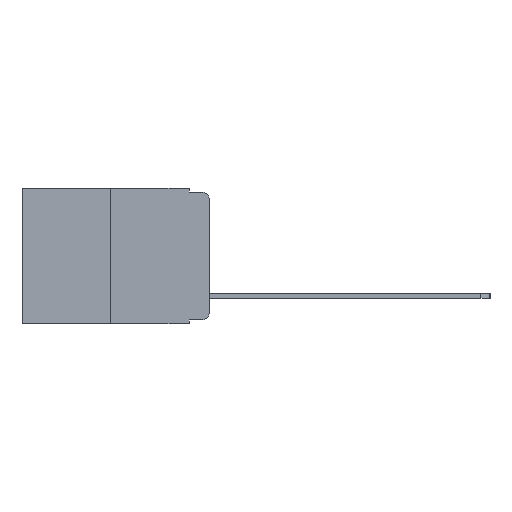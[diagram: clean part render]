
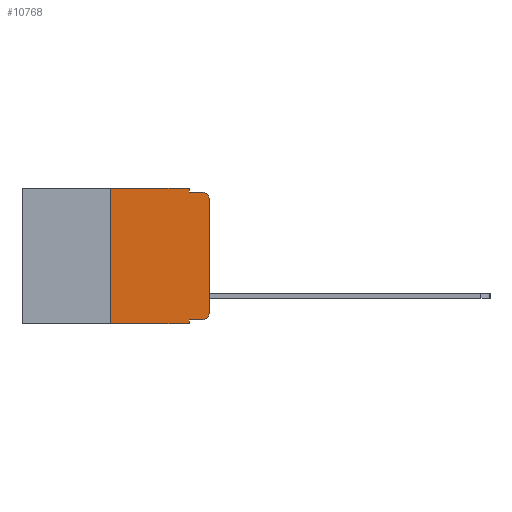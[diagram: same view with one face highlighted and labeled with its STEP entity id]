
A CAD part, left-side view. The second image highlights one B-rep face of the part: STEP entity #10768.
In plain terms, the highlighted planar face has unit normal (-1, 0, 0).
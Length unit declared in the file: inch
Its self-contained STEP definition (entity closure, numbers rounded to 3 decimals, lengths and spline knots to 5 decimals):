
#59 = EDGE_LOOP ( 'NONE', ( #7966, #12042, #20362, #16670, #18114, #4457, #2379, #17849, #21247, #2677 ) ) ;
#522 = CARTESIAN_POINT ( 'NONE',  ( 0., 0.25, -0.343 ) ) ;
#590 = CIRCLE ( 'NONE', #12441, 0.02 ) ;
#1751 = VERTEX_POINT ( 'NONE', #12122 ) ;
#2349 = VERTEX_POINT ( 'NONE', #16459 ) ;
#2371 = DIRECTION ( 'NONE',  ( 0., -1., 0. ) ) ;
#2379 = ORIENTED_EDGE ( 'NONE', *, *, #17304, .T. ) ;
#2425 = VERTEX_POINT ( 'NONE', #12521 ) ;
#2677 = ORIENTED_EDGE ( 'NONE', *, *, #8130, .T. ) ;
#2835 = EDGE_CURVE ( 'NONE', #20767, #2425, #19707, .T. ) ;
#3055 = CARTESIAN_POINT ( 'NONE',  ( 0., 0.02, -0.03 ) ) ;
#3078 = EDGE_CURVE ( 'NONE', #16209, #1751, #15110, .T. ) ;
#3183 = LINE ( 'NONE', #14919, #12591 ) ;
#3663 = VECTOR ( 'NONE', #22484, 39.37008 ) ;
#4039 = CARTESIAN_POINT ( 'NONE',  ( 0., 0.473, -0.343 ) ) ;
#4457 = ORIENTED_EDGE ( 'NONE', *, *, #2835, .F. ) ;
#4600 = CARTESIAN_POINT ( 'NONE',  ( 0., 0.051, -0.343 ) ) ;
#4985 = DIRECTION ( 'NONE',  ( 0., 0., -1. ) ) ;
#5203 = FACE_OUTER_BOUND ( 'NONE', #59, .T. ) ;
#6213 = DIRECTION ( 'NONE',  ( 0., 0., 1. ) ) ;
#6224 = EDGE_CURVE ( 'NONE', #16209, #16141, #14767, .T. ) ;
#6376 = VECTOR ( 'NONE', #8474, 39.37008 ) ;
#7515 = LINE ( 'NONE', #13726, #12458 ) ;
#7887 = AXIS2_PLACEMENT_3D ( 'NONE', #3055, #16147, #4985 ) ;
#7966 = ORIENTED_EDGE ( 'NONE', *, *, #11653, .T. ) ;
#8130 = EDGE_CURVE ( 'NONE', #1751, #2349, #590, .T. ) ;
#8420 = CARTESIAN_POINT ( 'NONE',  ( 0., 0., 0. ) ) ;
#8424 = VERTEX_POINT ( 'NONE', #8442 ) ;
#8442 = CARTESIAN_POINT ( 'NONE',  ( 0., 0.051, 0. ) ) ;
#8474 = DIRECTION ( 'NONE',  ( 0., -1., 0. ) ) ;
#8501 = DIRECTION ( 'NONE',  ( 0., 0., -1. ) ) ;
#8521 = VECTOR ( 'NONE', #2371, 39.37008 ) ;
#8726 = EDGE_CURVE ( 'NONE', #8424, #23268, #3183, .T. ) ;
#8734 = LINE ( 'NONE', #8420, #22222 ) ;
#8911 = EDGE_CURVE ( 'NONE', #23268, #14359, #23161, .T. ) ;
#9411 = CIRCLE ( 'NONE', #7887, 0.02 ) ;
#9768 = CARTESIAN_POINT ( 'NONE',  ( 0., 0.051, -0.01 ) ) ;
#9835 = VERTEX_POINT ( 'NONE', #23696 ) ;
#10120 = CARTESIAN_POINT ( 'NONE',  ( 0., 0.02, -0.313 ) ) ;
#10267 = PLANE ( 'NONE',  #13579 ) ;
#10768 = ADVANCED_FACE ( 'NONE', ( #5203 ), #10267, .F. ) ;
#11653 = EDGE_CURVE ( 'NONE', #2349, #9835, #8734, .T. ) ;
#12000 = DIRECTION ( 'NONE',  ( 0., 0., -1. ) ) ;
#12042 = ORIENTED_EDGE ( 'NONE', *, *, #14939, .T. ) ;
#12122 = CARTESIAN_POINT ( 'NONE',  ( 0., 0.02, -0.333 ) ) ;
#12218 = DIRECTION ( 'NONE',  ( 0., 0., 1. ) ) ;
#12441 = AXIS2_PLACEMENT_3D ( 'NONE', #10120, #22970, #12000 ) ;
#12458 = VECTOR ( 'NONE', #15592, 39.37008 ) ;
#12521 = CARTESIAN_POINT ( 'NONE',  ( 0., 0.25, 0. ) ) ;
#12591 = VECTOR ( 'NONE', #16758, 39.37008 ) ;
#13579 = AXIS2_PLACEMENT_3D ( 'NONE', #13945, #19536, #8501 ) ;
#13644 = DIRECTION ( 'NONE',  ( 0., 0., -1. ) ) ;
#13726 = CARTESIAN_POINT ( 'NONE',  ( 0., 0.473, 0. ) ) ;
#13945 = CARTESIAN_POINT ( 'NONE',  ( 0., 0.473, 0. ) ) ;
#14359 = VERTEX_POINT ( 'NONE', #17921 ) ;
#14767 = LINE ( 'NONE', #17242, #19042 ) ;
#14919 = CARTESIAN_POINT ( 'NONE',  ( 0., 0.051, 0. ) ) ;
#14939 = EDGE_CURVE ( 'NONE', #9835, #14359, #9411, .T. ) ;
#15110 = LINE ( 'NONE', #18303, #6376 ) ;
#15592 = DIRECTION ( 'NONE',  ( 0., -1., 0. ) ) ;
#16005 = CARTESIAN_POINT ( 'NONE',  ( 0., 0.051, -0.333 ) ) ;
#16141 = VERTEX_POINT ( 'NONE', #4600 ) ;
#16147 = DIRECTION ( 'NONE',  ( -1., 0., 0. ) ) ;
#16209 = VERTEX_POINT ( 'NONE', #16005 ) ;
#16459 = CARTESIAN_POINT ( 'NONE',  ( 0., 0., -0.313 ) ) ;
#16651 = EDGE_CURVE ( 'NONE', #2425, #8424, #7515, .T. ) ;
#16670 = ORIENTED_EDGE ( 'NONE', *, *, #8726, .F. ) ;
#16758 = DIRECTION ( 'NONE',  ( 0., 0., -1. ) ) ;
#16946 = CARTESIAN_POINT ( 'NONE',  ( 0., 0.051, -0.01 ) ) ;
#17242 = CARTESIAN_POINT ( 'NONE',  ( 0., 0.051, 0. ) ) ;
#17304 = EDGE_CURVE ( 'NONE', #20767, #16141, #23915, .T. ) ;
#17849 = ORIENTED_EDGE ( 'NONE', *, *, #6224, .F. ) ;
#17921 = CARTESIAN_POINT ( 'NONE',  ( 0., 0.02, -0.01 ) ) ;
#18114 = ORIENTED_EDGE ( 'NONE', *, *, #16651, .F. ) ;
#18303 = CARTESIAN_POINT ( 'NONE',  ( 0., 0.051, -0.333 ) ) ;
#19042 = VECTOR ( 'NONE', #13644, 39.37008 ) ;
#19536 = DIRECTION ( 'NONE',  ( 1., 0., 0. ) ) ;
#19599 = CARTESIAN_POINT ( 'NONE',  ( 0., 0.25, 0. ) ) ;
#19707 = LINE ( 'NONE', #19599, #23975 ) ;
#20362 = ORIENTED_EDGE ( 'NONE', *, *, #8911, .F. ) ;
#20767 = VERTEX_POINT ( 'NONE', #522 ) ;
#21247 = ORIENTED_EDGE ( 'NONE', *, *, #3078, .T. ) ;
#22222 = VECTOR ( 'NONE', #12218, 39.37008 ) ;
#22484 = DIRECTION ( 'NONE',  ( 0., -1., 0. ) ) ;
#22970 = DIRECTION ( 'NONE',  ( -1., 0., 0. ) ) ;
#23161 = LINE ( 'NONE', #9768, #8521 ) ;
#23268 = VERTEX_POINT ( 'NONE', #16946 ) ;
#23696 = CARTESIAN_POINT ( 'NONE',  ( 0., 0., -0.03 ) ) ;
#23915 = LINE ( 'NONE', #4039, #3663 ) ;
#23975 = VECTOR ( 'NONE', #6213, 39.37008 ) ;
